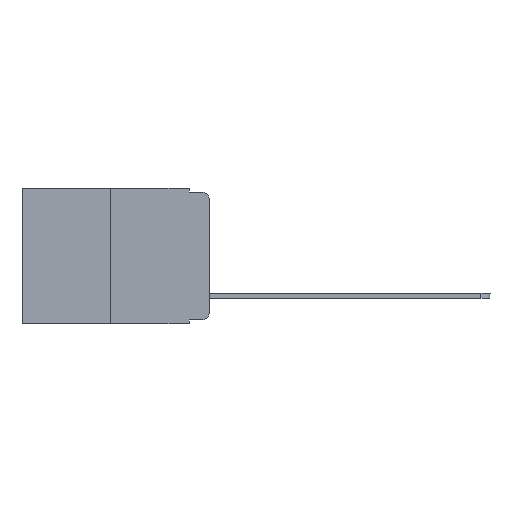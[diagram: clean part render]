
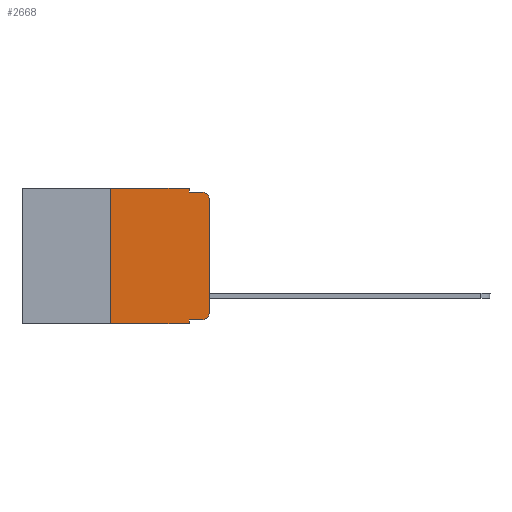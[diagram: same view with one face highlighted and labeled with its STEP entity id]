
A CAD part, left-side view. The second image highlights one B-rep face of the part: STEP entity #2668.
In plain terms, the highlighted planar face has unit normal (-1, 0, 0).
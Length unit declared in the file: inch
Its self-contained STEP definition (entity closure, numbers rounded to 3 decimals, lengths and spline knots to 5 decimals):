
#317 = DIRECTION ( 'NONE',  ( -1., 0., 0. ) ) ;
#358 = ORIENTED_EDGE ( 'NONE', *, *, #7459, .T. ) ;
#402 = ORIENTED_EDGE ( 'NONE', *, *, #2294, .T. ) ;
#863 = ORIENTED_EDGE ( 'NONE', *, *, #3320, .F. ) ;
#881 = CARTESIAN_POINT ( 'NONE',  ( 0., 0.473, -0.343 ) ) ;
#1147 = LINE ( 'NONE', #3301, #3561 ) ;
#1154 = CARTESIAN_POINT ( 'NONE',  ( 0., 0.02, -0.313 ) ) ;
#1240 = DIRECTION ( 'NONE',  ( -1., 0., 0. ) ) ;
#1257 = LINE ( 'NONE', #3370, #1499 ) ;
#1288 = LINE ( 'NONE', #881, #4943 ) ;
#1499 = VECTOR ( 'NONE', #6449, 39.37008 ) ;
#1529 = CARTESIAN_POINT ( 'NONE',  ( 0., 0.02, -0.01 ) ) ;
#1775 = EDGE_CURVE ( 'NONE', #5977, #8705, #2127, .T. ) ;
#1798 = EDGE_CURVE ( 'NONE', #7877, #3378, #8036, .T. ) ;
#1907 = CARTESIAN_POINT ( 'NONE',  ( 0., 0.051, -0.01 ) ) ;
#1947 = ORIENTED_EDGE ( 'NONE', *, *, #1798, .F. ) ;
#2076 = AXIS2_PLACEMENT_3D ( 'NONE', #7761, #4640, #8526 ) ;
#2127 = CIRCLE ( 'NONE', #3899, 0.02 ) ;
#2294 = EDGE_CURVE ( 'NONE', #7877, #5977, #8160, .T. ) ;
#2443 = ORIENTED_EDGE ( 'NONE', *, *, #5687, .F. ) ;
#2533 = DIRECTION ( 'NONE',  ( 0., -1., 0. ) ) ;
#2668 = ADVANCED_FACE ( 'NONE', ( #3818 ), #6858, .F. ) ;
#2673 = VERTEX_POINT ( 'NONE', #6232 ) ;
#3188 = CARTESIAN_POINT ( 'NONE',  ( 0., 0.02, -0.333 ) ) ;
#3193 = EDGE_CURVE ( 'NONE', #8705, #6415, #1257, .T. ) ;
#3301 = CARTESIAN_POINT ( 'NONE',  ( 0., 0.051, 0. ) ) ;
#3320 = EDGE_CURVE ( 'NONE', #2673, #8360, #8263, .T. ) ;
#3370 = CARTESIAN_POINT ( 'NONE',  ( 0., 0., 0. ) ) ;
#3378 = VERTEX_POINT ( 'NONE', #6654 ) ;
#3561 = VECTOR ( 'NONE', #8763, 39.37008 ) ;
#3581 = CARTESIAN_POINT ( 'NONE',  ( 0., 0.25, 0. ) ) ;
#3654 = AXIS2_PLACEMENT_3D ( 'NONE', #5779, #1240, #8826 ) ;
#3690 = LINE ( 'NONE', #6478, #6576 ) ;
#3793 = DIRECTION ( 'NONE',  ( 0., -1., 0. ) ) ;
#3818 = FACE_OUTER_BOUND ( 'NONE', #6429, .T. ) ;
#3899 = AXIS2_PLACEMENT_3D ( 'NONE', #1154, #317, #5790 ) ;
#4037 = EDGE_CURVE ( 'NONE', #8685, #8724, #3690, .T. ) ;
#4077 = EDGE_CURVE ( 'NONE', #8724, #2673, #1147, .T. ) ;
#4094 = VECTOR ( 'NONE', #7372, 39.37008 ) ;
#4276 = DIRECTION ( 'NONE',  ( 0., -1., 0. ) ) ;
#4499 = ORIENTED_EDGE ( 'NONE', *, *, #4037, .F. ) ;
#4640 = DIRECTION ( 'NONE',  ( 1., 0., 0. ) ) ;
#4683 = DIRECTION ( 'NONE',  ( 0., -1., 0. ) ) ;
#4883 = ORIENTED_EDGE ( 'NONE', *, *, #3193, .T. ) ;
#4943 = VECTOR ( 'NONE', #4683, 39.37008 ) ;
#5128 = CARTESIAN_POINT ( 'NONE',  ( 0., 0.051, 0. ) ) ;
#5349 = VERTEX_POINT ( 'NONE', #6794 ) ;
#5687 = EDGE_CURVE ( 'NONE', #5349, #8685, #9071, .T. ) ;
#5779 = CARTESIAN_POINT ( 'NONE',  ( 0., 0.02, -0.03 ) ) ;
#5784 = CARTESIAN_POINT ( 'NONE',  ( 0., 0.25, 0. ) ) ;
#5790 = DIRECTION ( 'NONE',  ( 0., 0., -1. ) ) ;
#5894 = CARTESIAN_POINT ( 'NONE',  ( 0., 0., -0.313 ) ) ;
#5977 = VERTEX_POINT ( 'NONE', #3188 ) ;
#6230 = VECTOR ( 'NONE', #3793, 39.37008 ) ;
#6232 = CARTESIAN_POINT ( 'NONE',  ( 0., 0.051, -0.01 ) ) ;
#6415 = VERTEX_POINT ( 'NONE', #6494 ) ;
#6429 = EDGE_LOOP ( 'NONE', ( #4883, #358, #863, #7918, #4499, #2443, #9307, #1947, #402, #8539 ) ) ;
#6449 = DIRECTION ( 'NONE',  ( 0., 0., 1. ) ) ;
#6478 = CARTESIAN_POINT ( 'NONE',  ( 0., 0.473, 0. ) ) ;
#6494 = CARTESIAN_POINT ( 'NONE',  ( 0., 0., -0.03 ) ) ;
#6576 = VECTOR ( 'NONE', #2533, 39.37008 ) ;
#6654 = CARTESIAN_POINT ( 'NONE',  ( 0., 0.051, -0.343 ) ) ;
#6794 = CARTESIAN_POINT ( 'NONE',  ( 0., 0.25, -0.343 ) ) ;
#6837 = CARTESIAN_POINT ( 'NONE',  ( 0., 0.051, -0.333 ) ) ;
#6858 = PLANE ( 'NONE',  #2076 ) ;
#7032 = VECTOR ( 'NONE', #9742, 39.37008 ) ;
#7183 = VECTOR ( 'NONE', #4276, 39.37008 ) ;
#7372 = DIRECTION ( 'NONE',  ( 0., 0., -1. ) ) ;
#7459 = EDGE_CURVE ( 'NONE', #6415, #8360, #9892, .T. ) ;
#7761 = CARTESIAN_POINT ( 'NONE',  ( 0., 0.473, 0. ) ) ;
#7877 = VERTEX_POINT ( 'NONE', #8717 ) ;
#7918 = ORIENTED_EDGE ( 'NONE', *, *, #4077, .F. ) ;
#8036 = LINE ( 'NONE', #9610, #4094 ) ;
#8160 = LINE ( 'NONE', #6837, #6230 ) ;
#8263 = LINE ( 'NONE', #1907, #7183 ) ;
#8360 = VERTEX_POINT ( 'NONE', #1529 ) ;
#8526 = DIRECTION ( 'NONE',  ( 0., 0., -1. ) ) ;
#8539 = ORIENTED_EDGE ( 'NONE', *, *, #1775, .T. ) ;
#8685 = VERTEX_POINT ( 'NONE', #3581 ) ;
#8705 = VERTEX_POINT ( 'NONE', #5894 ) ;
#8717 = CARTESIAN_POINT ( 'NONE',  ( 0., 0.051, -0.333 ) ) ;
#8724 = VERTEX_POINT ( 'NONE', #5128 ) ;
#8763 = DIRECTION ( 'NONE',  ( 0., 0., -1. ) ) ;
#8826 = DIRECTION ( 'NONE',  ( 0., 0., -1. ) ) ;
#9071 = LINE ( 'NONE', #5784, #7032 ) ;
#9087 = EDGE_CURVE ( 'NONE', #5349, #3378, #1288, .T. ) ;
#9307 = ORIENTED_EDGE ( 'NONE', *, *, #9087, .T. ) ;
#9610 = CARTESIAN_POINT ( 'NONE',  ( 0., 0.051, 0. ) ) ;
#9742 = DIRECTION ( 'NONE',  ( 0., 0., 1. ) ) ;
#9892 = CIRCLE ( 'NONE', #3654, 0.02 ) ;
